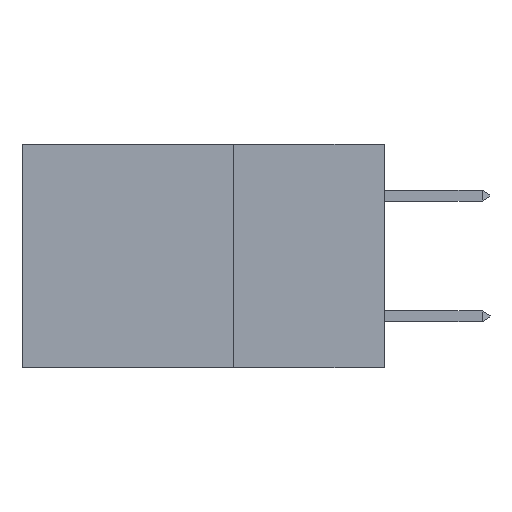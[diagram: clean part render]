
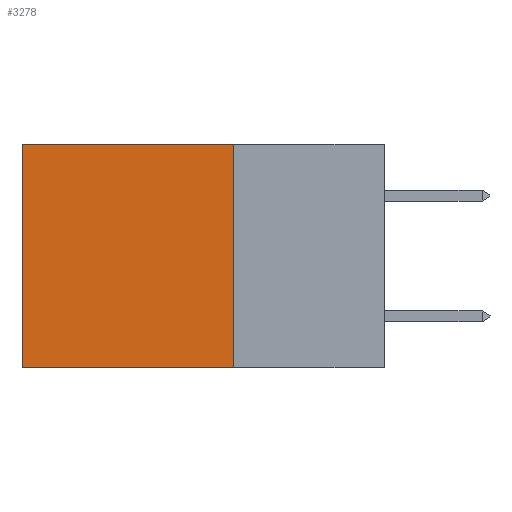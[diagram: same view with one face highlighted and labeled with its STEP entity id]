
A CAD part, left-side view. The second image highlights one B-rep face of the part: STEP entity #3278.
In plain terms, the highlighted planar face has unit normal (-1, 0, 0).
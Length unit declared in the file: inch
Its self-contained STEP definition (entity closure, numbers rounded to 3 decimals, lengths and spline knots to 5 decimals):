
#509 = EDGE_LOOP ( 'NONE', ( #3400, #30009, #5661, #8231 ) ) ;
#936 = CARTESIAN_POINT ( 'NONE',  ( 0.2875, 0.6, -0.37 ) ) ;
#1145 = DIRECTION ( 'NONE',  ( 0., 0., -1. ) ) ;
#2457 = VERTEX_POINT ( 'NONE', #936 ) ;
#3278 = ADVANCED_FACE ( 'NONE', ( #29072 ), #5271, .F. ) ;
#3400 = ORIENTED_EDGE ( 'NONE', *, *, #7795, .T. ) ;
#4714 = DIRECTION ( 'NONE',  ( 0., 0., -1. ) ) ;
#4883 = CARTESIAN_POINT ( 'NONE',  ( 0.2875, 0.6, 0. ) ) ;
#5271 = PLANE ( 'NONE',  #9743 ) ;
#5612 = DIRECTION ( 'NONE',  ( 1., 0., 0. ) ) ;
#5661 = ORIENTED_EDGE ( 'NONE', *, *, #31986, .F. ) ;
#7795 = EDGE_CURVE ( 'NONE', #29996, #2457, #18284, .T. ) ;
#8231 = ORIENTED_EDGE ( 'NONE', *, *, #25335, .T. ) ;
#8290 = LINE ( 'NONE', #29795, #14515 ) ;
#8910 = CARTESIAN_POINT ( 'NONE',  ( 0.2875, 0.25, 0. ) ) ;
#9743 = AXIS2_PLACEMENT_3D ( 'NONE', #21486, #5612, #29418 ) ;
#9838 = CARTESIAN_POINT ( 'NONE',  ( 0.2875, 0.25, 0. ) ) ;
#10747 = VECTOR ( 'NONE', #26048, 39.37008 ) ;
#12968 = CARTESIAN_POINT ( 'NONE',  ( 0.2875, 0.25, -0.37 ) ) ;
#13819 = VECTOR ( 'NONE', #1145, 39.37008 ) ;
#14515 = VECTOR ( 'NONE', #16396, 39.37008 ) ;
#16068 = VERTEX_POINT ( 'NONE', #23697 ) ;
#16396 = DIRECTION ( 'NONE',  ( 0., 1., 0. ) ) ;
#16859 = EDGE_CURVE ( 'NONE', #22317, #2457, #8290, .T. ) ;
#18284 = LINE ( 'NONE', #4883, #31165 ) ;
#18766 = LINE ( 'NONE', #9838, #10747 ) ;
#20263 = CARTESIAN_POINT ( 'NONE',  ( 0.2875, 0.6, 0. ) ) ;
#21486 = CARTESIAN_POINT ( 'NONE',  ( 0.2875, 0.25, 0. ) ) ;
#22317 = VERTEX_POINT ( 'NONE', #12968 ) ;
#23697 = CARTESIAN_POINT ( 'NONE',  ( 0.2875, 0.25, 0. ) ) ;
#25335 = EDGE_CURVE ( 'NONE', #16068, #29996, #18766, .T. ) ;
#26048 = DIRECTION ( 'NONE',  ( 0., 1., 0. ) ) ;
#28283 = LINE ( 'NONE', #8910, #13819 ) ;
#29072 = FACE_OUTER_BOUND ( 'NONE', #509, .T. ) ;
#29418 = DIRECTION ( 'NONE',  ( 0., 0., -1. ) ) ;
#29795 = CARTESIAN_POINT ( 'NONE',  ( 0.2875, 0.25, -0.37 ) ) ;
#29996 = VERTEX_POINT ( 'NONE', #20263 ) ;
#30009 = ORIENTED_EDGE ( 'NONE', *, *, #16859, .F. ) ;
#31165 = VECTOR ( 'NONE', #4714, 39.37008 ) ;
#31986 = EDGE_CURVE ( 'NONE', #16068, #22317, #28283, .T. ) ;
